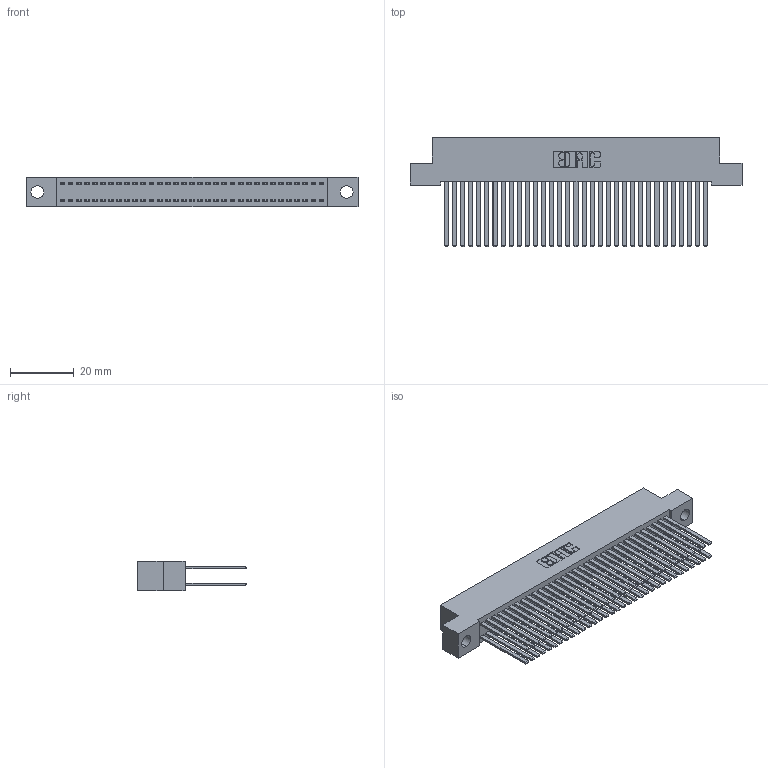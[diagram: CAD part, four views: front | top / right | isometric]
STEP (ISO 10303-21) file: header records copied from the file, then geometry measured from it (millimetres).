
FILE_DESCRIPTION (( 'STEP AP203' ), '1' );
FILE_NAME ('392-066-544-204.STEP', '2019-10-09T11:17:42', ( '' ), ( '' ), 'SwSTEP 2.0', 'SolidWorks 2016', '' );
FILE_SCHEMA (( 'CONFIG_CONTROL_DESIGN' ));
Length unit declared in the file: inch
Products named in the file (3): 342 Part_.156 TH; 345-292-001_345-293-144; 392-066-544-204
Assembly tree (67 placements, depth 2):
  392-066-544-204
    342 Part_.156 TH
    345-292-001_345-293-144  x66
Bounding box: 104.14 x 34.3 x 9.4 mm (x, y, z)
Volume: 10152.5 mm3; surface area: 18690.4 mm2
Topology: 67 solids, 67 shells, 3146 faces, 9341 edges, 6138 vertices
Faces by surface type: plane 2178, cylinder 968
Entity records: 22081 total; most frequent: CARTESIAN_POINT 3666, ORIENTED_EDGE 3602, DIRECTION 3145, EDGE_CURVE 1801, VECTOR 1677, LINE 1677, VERTEX_POINT 1198, AXIS2_PLACEMENT_3D 734
